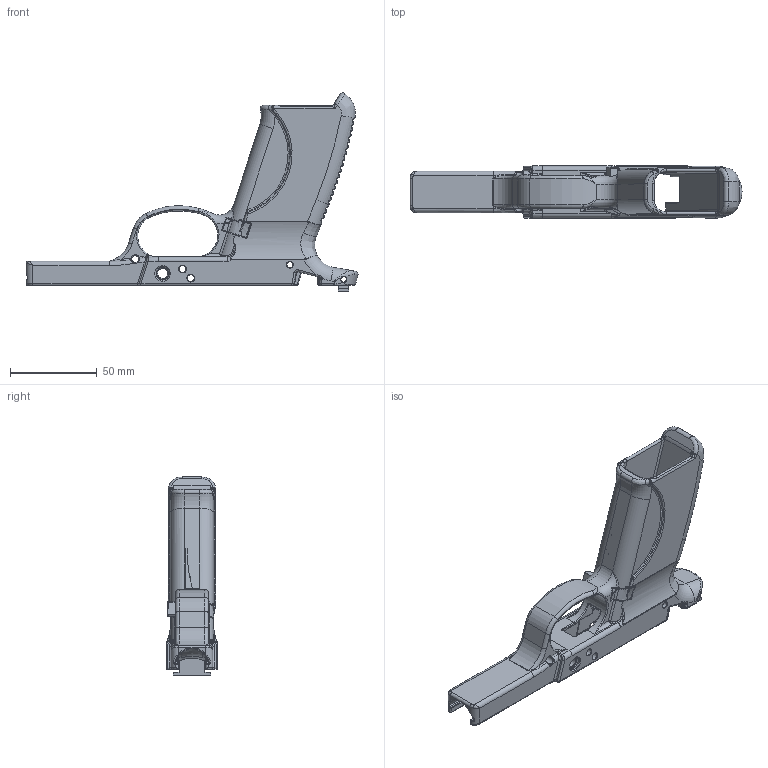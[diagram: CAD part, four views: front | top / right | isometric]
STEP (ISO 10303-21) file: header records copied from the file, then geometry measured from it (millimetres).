
FILE_DESCRIPTION(/* description */ (''),/* implementation_level */ '2;1');
FILE_NAME(/* name */ '0bd4680d-a830-4799-83d2-aa42fbc88a1e.stp',/* time_stamp */ '2019-06-02T13:09:54-04:00',/* author */ ('suzuki450ltr'),/* organization */ (''),/* preprocessor_version */ 'ST-DEVELOPER v18',/* originating_system */ 'Autodesk Translation Framework v8.2.0.1029',/* authorisation */ '');
FILE_SCHEMA (('AUTOMOTIVE_DESIGN { 1 0 10303 214 3 1 1 }'));
Products named in the file (3): SR9; Mag Catch SR9; SR9 Rear Rail
Assembly tree (2 placements, depth 2):
  SR9
    Mag Catch SR9
    SR9 Rear Rail
Bounding box: 191.67 x 30 x 114.42 mm (x, y, z)
Volume: 81192.7 mm3; surface area: 50857.8 mm2
Topology: 3 solids, 3 shells, 1460 faces, 3482 edges, 1927 vertices
Faces by surface type: cylinder 516, bspline 481, plane 205, torus 186, sphere 37, cone 35
Full cylindrical faces by diameter (mm): 3.175 x3, 3.5 x1, 4 x6, 4.36 x1, 5.8 x2, 8 x1
Entity records: 58516 total; most frequent: CARTESIAN_POINT 27198, ORIENTED_EDGE 6794, DIRECTION 6214, EDGE_CURVE 3397, AXIS2_PLACEMENT_3D 2555, VERTEX_POINT 1928, EDGE_LOOP 1481, FACE_OUTER_BOUND 1460
